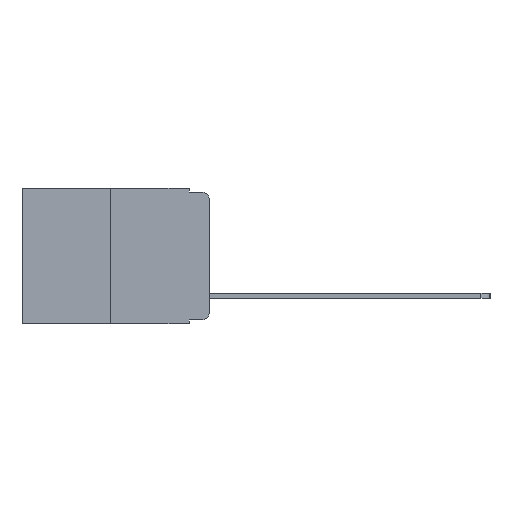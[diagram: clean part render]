
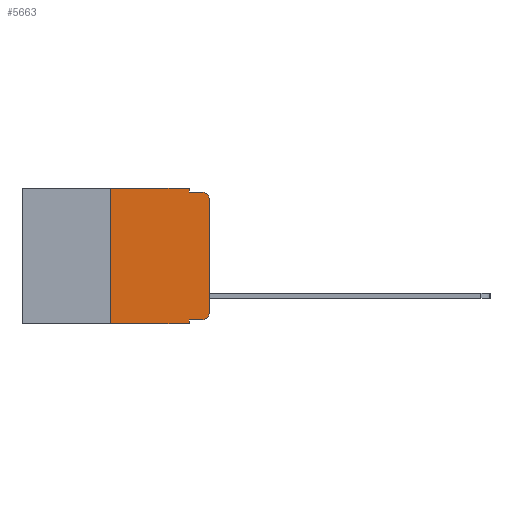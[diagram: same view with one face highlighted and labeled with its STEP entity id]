
A CAD part, left-side view. The second image highlights one B-rep face of the part: STEP entity #5663.
In plain terms, the highlighted planar face has unit normal (-1, 0, 0).
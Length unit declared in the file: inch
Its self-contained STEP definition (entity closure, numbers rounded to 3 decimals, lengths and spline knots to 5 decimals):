
#342 = CARTESIAN_POINT ( 'NONE',  ( 0., 0.051, -0.343 ) ) ;
#651 = CARTESIAN_POINT ( 'NONE',  ( 0., 0., -0.313 ) ) ;
#672 = EDGE_CURVE ( 'NONE', #13326, #1751, #10366, .T. ) ;
#1169 = CARTESIAN_POINT ( 'NONE',  ( 0., 0.473, 0. ) ) ;
#1195 = ORIENTED_EDGE ( 'NONE', *, *, #13681, .F. ) ;
#1644 = ORIENTED_EDGE ( 'NONE', *, *, #1907, .T. ) ;
#1751 = VERTEX_POINT ( 'NONE', #9414 ) ;
#1907 = EDGE_CURVE ( 'NONE', #5249, #13761, #8774, .T. ) ;
#2068 = FACE_OUTER_BOUND ( 'NONE', #7738, .T. ) ;
#2231 = DIRECTION ( 'NONE',  ( 1., 0., 0. ) ) ;
#2319 = DIRECTION ( 'NONE',  ( -1., 0., 0. ) ) ;
#2940 = VERTEX_POINT ( 'NONE', #8388 ) ;
#3022 = AXIS2_PLACEMENT_3D ( 'NONE', #11045, #2319, #12465 ) ;
#3207 = DIRECTION ( 'NONE',  ( 0., -1., 0. ) ) ;
#3742 = ORIENTED_EDGE ( 'NONE', *, *, #15566, .F. ) ;
#3820 = CARTESIAN_POINT ( 'NONE',  ( 0., 0.051, 0. ) ) ;
#3916 = CARTESIAN_POINT ( 'NONE',  ( 0., 0.051, 0. ) ) ;
#4406 = CARTESIAN_POINT ( 'NONE',  ( 0., 0.051, -0.333 ) ) ;
#4599 = VECTOR ( 'NONE', #12561, 39.37008 ) ;
#4612 = CARTESIAN_POINT ( 'NONE',  ( 0., 0.25, 0. ) ) ;
#4735 = VERTEX_POINT ( 'NONE', #6939 ) ;
#5108 = LINE ( 'NONE', #4612, #12291 ) ;
#5128 = LINE ( 'NONE', #4406, #8541 ) ;
#5249 = VERTEX_POINT ( 'NONE', #15370 ) ;
#5328 = CARTESIAN_POINT ( 'NONE',  ( 0., 0.051, -0.333 ) ) ;
#5663 = ADVANCED_FACE ( 'NONE', ( #2068 ), #17971, .F. ) ;
#6144 = CIRCLE ( 'NONE', #3022, 0.02 ) ;
#6379 = DIRECTION ( 'NONE',  ( -1., 0., 0. ) ) ;
#6644 = VECTOR ( 'NONE', #9404, 39.37008 ) ;
#6799 = VERTEX_POINT ( 'NONE', #13356 ) ;
#6939 = CARTESIAN_POINT ( 'NONE',  ( 0., 0.25, 0. ) ) ;
#7738 = EDGE_LOOP ( 'NONE', ( #10542, #14336, #3742, #8128, #15646, #1195, #1644, #9431, #13230, #13679 ) ) ;
#7993 = LINE ( 'NONE', #16460, #6644 ) ;
#8035 = LINE ( 'NONE', #3916, #4599 ) ;
#8128 = ORIENTED_EDGE ( 'NONE', *, *, #14623, .F. ) ;
#8388 = CARTESIAN_POINT ( 'NONE',  ( 0., 0.02, -0.333 ) ) ;
#8541 = VECTOR ( 'NONE', #13013, 39.37008 ) ;
#8774 = LINE ( 'NONE', #11889, #12565 ) ;
#8903 = EDGE_CURVE ( 'NONE', #2940, #13326, #6144, .T. ) ;
#8910 = VERTEX_POINT ( 'NONE', #5328 ) ;
#8973 = DIRECTION ( 'NONE',  ( 0., 0., 1. ) ) ;
#9404 = DIRECTION ( 'NONE',  ( 0., -1., 0. ) ) ;
#9414 = CARTESIAN_POINT ( 'NONE',  ( 0., 0., -0.03 ) ) ;
#9431 = ORIENTED_EDGE ( 'NONE', *, *, #10825, .F. ) ;
#9853 = EDGE_CURVE ( 'NONE', #8910, #2940, #5128, .T. ) ;
#10325 = CIRCLE ( 'NONE', #15309, 0.02 ) ;
#10366 = LINE ( 'NONE', #10533, #14163 ) ;
#10533 = CARTESIAN_POINT ( 'NONE',  ( 0., 0., 0. ) ) ;
#10542 = ORIENTED_EDGE ( 'NONE', *, *, #672, .T. ) ;
#10637 = AXIS2_PLACEMENT_3D ( 'NONE', #10973, #2231, #12392 ) ;
#10825 = EDGE_CURVE ( 'NONE', #8910, #13761, #17528, .T. ) ;
#10973 = CARTESIAN_POINT ( 'NONE',  ( 0., 0.473, 0. ) ) ;
#11045 = CARTESIAN_POINT ( 'NONE',  ( 0., 0.02, -0.313 ) ) ;
#11367 = DIRECTION ( 'NONE',  ( 0., -1., 0. ) ) ;
#11387 = VECTOR ( 'NONE', #13910, 39.37008 ) ;
#11889 = CARTESIAN_POINT ( 'NONE',  ( 0., 0.473, -0.343 ) ) ;
#12074 = LINE ( 'NONE', #1169, #12520 ) ;
#12291 = VECTOR ( 'NONE', #8973, 39.37008 ) ;
#12392 = DIRECTION ( 'NONE',  ( 0., 0., -1. ) ) ;
#12465 = DIRECTION ( 'NONE',  ( 0., 0., -1. ) ) ;
#12520 = VECTOR ( 'NONE', #11367, 39.37008 ) ;
#12561 = DIRECTION ( 'NONE',  ( 0., 0., -1. ) ) ;
#12565 = VECTOR ( 'NONE', #3207, 39.37008 ) ;
#12612 = DIRECTION ( 'NONE',  ( 0., 0., 1. ) ) ;
#13013 = DIRECTION ( 'NONE',  ( 0., -1., 0. ) ) ;
#13230 = ORIENTED_EDGE ( 'NONE', *, *, #9853, .T. ) ;
#13326 = VERTEX_POINT ( 'NONE', #651 ) ;
#13356 = CARTESIAN_POINT ( 'NONE',  ( 0., 0.051, 0. ) ) ;
#13472 = EDGE_CURVE ( 'NONE', #4735, #6799, #12074, .T. ) ;
#13679 = ORIENTED_EDGE ( 'NONE', *, *, #8903, .T. ) ;
#13681 = EDGE_CURVE ( 'NONE', #5249, #4735, #5108, .T. ) ;
#13761 = VERTEX_POINT ( 'NONE', #342 ) ;
#13910 = DIRECTION ( 'NONE',  ( 0., 0., -1. ) ) ;
#14163 = VECTOR ( 'NONE', #12612, 39.37008 ) ;
#14336 = ORIENTED_EDGE ( 'NONE', *, *, #18355, .T. ) ;
#14623 = EDGE_CURVE ( 'NONE', #6799, #15725, #8035, .T. ) ;
#14906 = CARTESIAN_POINT ( 'NONE',  ( 0., 0.02, -0.03 ) ) ;
#15185 = VERTEX_POINT ( 'NONE', #16657 ) ;
#15309 = AXIS2_PLACEMENT_3D ( 'NONE', #14906, #6379, #16308 ) ;
#15370 = CARTESIAN_POINT ( 'NONE',  ( 0., 0.25, -0.343 ) ) ;
#15422 = CARTESIAN_POINT ( 'NONE',  ( 0., 0.051, -0.01 ) ) ;
#15566 = EDGE_CURVE ( 'NONE', #15725, #15185, #7993, .T. ) ;
#15646 = ORIENTED_EDGE ( 'NONE', *, *, #13472, .F. ) ;
#15725 = VERTEX_POINT ( 'NONE', #15422 ) ;
#16308 = DIRECTION ( 'NONE',  ( 0., 0., -1. ) ) ;
#16460 = CARTESIAN_POINT ( 'NONE',  ( 0., 0.051, -0.01 ) ) ;
#16657 = CARTESIAN_POINT ( 'NONE',  ( 0., 0.02, -0.01 ) ) ;
#17528 = LINE ( 'NONE', #3820, #11387 ) ;
#17971 = PLANE ( 'NONE',  #10637 ) ;
#18355 = EDGE_CURVE ( 'NONE', #1751, #15185, #10325, .T. ) ;
